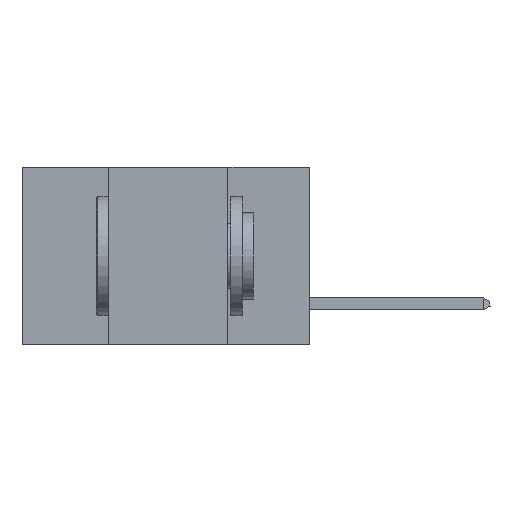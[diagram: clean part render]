
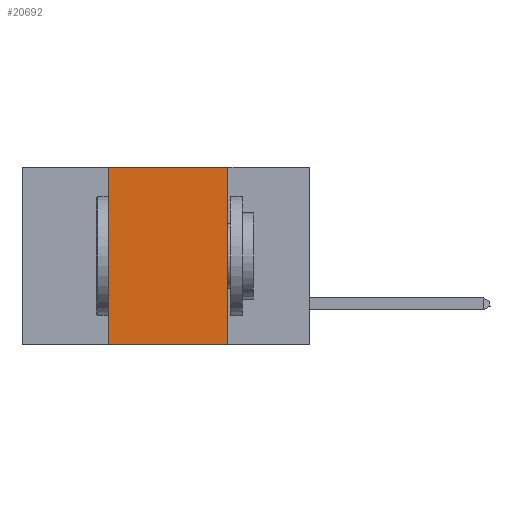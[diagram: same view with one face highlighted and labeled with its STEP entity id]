
A CAD part, left-side view. The second image highlights one B-rep face of the part: STEP entity #20692.
In plain terms, the highlighted planar face has unit normal (-1, 0, 0).
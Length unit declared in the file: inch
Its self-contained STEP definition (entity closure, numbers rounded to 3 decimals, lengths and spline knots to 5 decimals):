
#1278 = VECTOR ( 'NONE', #36699, 39.37008 ) ;
#2186 = DIRECTION ( 'NONE',  ( 0., 0., 1. ) ) ;
#4203 = LINE ( 'NONE', #40134, #38440 ) ;
#4998 = CARTESIAN_POINT ( 'NONE',  ( 0., 0.6, 0. ) ) ;
#6514 = CARTESIAN_POINT ( 'NONE',  ( 0., 0.6, 0. ) ) ;
#8531 = DIRECTION ( 'NONE',  ( 0., 0., -1. ) ) ;
#8726 = VERTEX_POINT ( 'NONE', #46228 ) ;
#11773 = ORIENTED_EDGE ( 'NONE', *, *, #32421, .F. ) ;
#13513 = DIRECTION ( 'NONE',  ( 0., -1., 0. ) ) ;
#14253 = CARTESIAN_POINT ( 'NONE',  ( 0., 0.42, -0.37 ) ) ;
#16713 = DIRECTION ( 'NONE',  ( 1., 0., 0. ) ) ;
#19699 = CARTESIAN_POINT ( 'NONE',  ( 0., 0.17, 0. ) ) ;
#20692 = ADVANCED_FACE ( 'NONE', ( #38529 ), #46973, .F. ) ;
#21492 = EDGE_CURVE ( 'NONE', #37424, #24771, #4203, .T. ) ;
#22048 = AXIS2_PLACEMENT_3D ( 'NONE', #4998, #16713, #8531 ) ;
#24145 = ORIENTED_EDGE ( 'NONE', *, *, #21492, .F. ) ;
#24771 = VERTEX_POINT ( 'NONE', #26905 ) ;
#26905 = CARTESIAN_POINT ( 'NONE',  ( 0., 0.42, 0. ) ) ;
#27458 = VECTOR ( 'NONE', #13513, 39.37008 ) ;
#28854 = EDGE_CURVE ( 'NONE', #32318, #8726, #49361, .T. ) ;
#31324 = LINE ( 'NONE', #6514, #1278 ) ;
#31906 = VECTOR ( 'NONE', #34298, 39.37008 ) ;
#32318 = VERTEX_POINT ( 'NONE', #36057 ) ;
#32421 = EDGE_CURVE ( 'NONE', #24771, #32318, #31324, .T. ) ;
#32508 = CARTESIAN_POINT ( 'NONE',  ( 0., 0.6, -0.37 ) ) ;
#34298 = DIRECTION ( 'NONE',  ( 0., 0., -1. ) ) ;
#36057 = CARTESIAN_POINT ( 'NONE',  ( 0., 0.17, 0. ) ) ;
#36699 = DIRECTION ( 'NONE',  ( 0., -1., 0. ) ) ;
#37424 = VERTEX_POINT ( 'NONE', #14253 ) ;
#37644 = LINE ( 'NONE', #32508, #27458 ) ;
#38440 = VECTOR ( 'NONE', #2186, 39.37008 ) ;
#38529 = FACE_OUTER_BOUND ( 'NONE', #45431, .T. ) ;
#38882 = ORIENTED_EDGE ( 'NONE', *, *, #42690, .T. ) ;
#40134 = CARTESIAN_POINT ( 'NONE',  ( 0., 0.42, 0. ) ) ;
#42690 = EDGE_CURVE ( 'NONE', #37424, #8726, #37644, .T. ) ;
#45431 = EDGE_LOOP ( 'NONE', ( #46064, #11773, #24145, #38882 ) ) ;
#46064 = ORIENTED_EDGE ( 'NONE', *, *, #28854, .F. ) ;
#46228 = CARTESIAN_POINT ( 'NONE',  ( 0., 0.17, -0.37 ) ) ;
#46973 = PLANE ( 'NONE',  #22048 ) ;
#49361 = LINE ( 'NONE', #19699, #31906 ) ;
